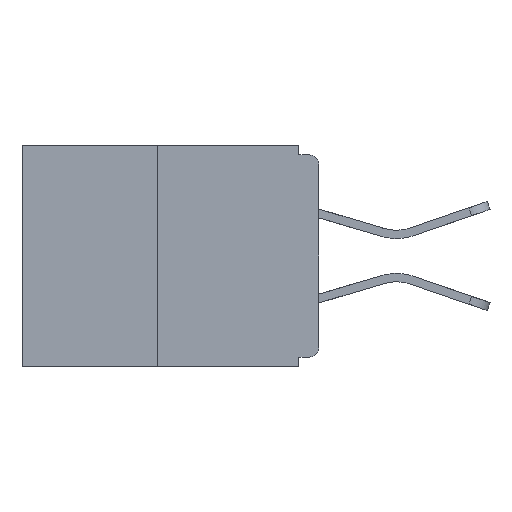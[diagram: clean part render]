
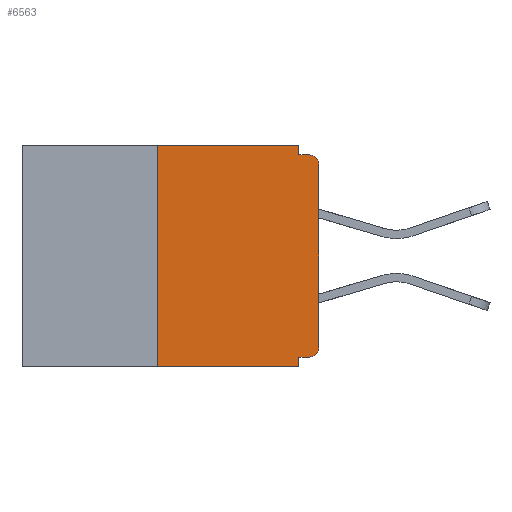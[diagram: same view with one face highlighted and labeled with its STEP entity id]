
A CAD part, left-side view. The second image highlights one B-rep face of the part: STEP entity #6563.
In plain terms, the highlighted planar face has unit normal (-1, 0, 0).
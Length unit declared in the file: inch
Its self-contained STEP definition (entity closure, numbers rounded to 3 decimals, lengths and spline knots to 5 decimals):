
#15 = VERTEX_POINT ( 'NONE', #8032 ) ;
#346 = EDGE_LOOP ( 'NONE', ( #6281, #9837, #14227, #1172, #9857, #2990, #5689, #12049, #8460, #6140 ) ) ;
#632 = VERTEX_POINT ( 'NONE', #10994 ) ;
#756 = VECTOR ( 'NONE', #11183, 39.37008 ) ;
#832 = CARTESIAN_POINT ( 'NONE',  ( 0., 0.25, 0. ) ) ;
#972 = AXIS2_PLACEMENT_3D ( 'NONE', #11592, #3609, #3659 ) ;
#1172 = ORIENTED_EDGE ( 'NONE', *, *, #12081, .F. ) ;
#1865 = DIRECTION ( 'NONE',  ( 0., 0., 1. ) ) ;
#2421 = DIRECTION ( 'NONE',  ( 0., 0., -1. ) ) ;
#2619 = CARTESIAN_POINT ( 'NONE',  ( 0., 0.46, 0. ) ) ;
#2790 = CARTESIAN_POINT ( 'NONE',  ( 0., 0., -0.015 ) ) ;
#2919 = DIRECTION ( 'NONE',  ( 0., 0., -1. ) ) ;
#2990 = ORIENTED_EDGE ( 'NONE', *, *, #7200, .T. ) ;
#3054 = CARTESIAN_POINT ( 'NONE',  ( 0., 0.031, -0.343 ) ) ;
#3356 = VECTOR ( 'NONE', #10710, 39.37008 ) ;
#3609 = DIRECTION ( 'NONE',  ( -1., 0., 0. ) ) ;
#3659 = DIRECTION ( 'NONE',  ( 0., 0., -1. ) ) ;
#4437 = CARTESIAN_POINT ( 'NONE',  ( 0., 0., -0.328 ) ) ;
#4690 = VECTOR ( 'NONE', #11553, 39.37008 ) ;
#4757 = CARTESIAN_POINT ( 'NONE',  ( 0., 0.031, 0. ) ) ;
#4964 = CARTESIAN_POINT ( 'NONE',  ( 0., 0.25, 0. ) ) ;
#5060 = LINE ( 'NONE', #3054, #14374 ) ;
#5541 = DIRECTION ( 'NONE',  ( 0., 0., -1. ) ) ;
#5686 = FACE_OUTER_BOUND ( 'NONE', #346, .T. ) ;
#5689 = ORIENTED_EDGE ( 'NONE', *, *, #9152, .T. ) ;
#5691 = LINE ( 'NONE', #4437, #756 ) ;
#6051 = LINE ( 'NONE', #13934, #4690 ) ;
#6140 = ORIENTED_EDGE ( 'NONE', *, *, #9027, .F. ) ;
#6281 = ORIENTED_EDGE ( 'NONE', *, *, #13015, .F. ) ;
#6563 = ADVANCED_FACE ( 'NONE', ( #5686 ), #8197, .F. ) ;
#6576 = EDGE_CURVE ( 'NONE', #11286, #8579, #7793, .T. ) ;
#6597 = VECTOR ( 'NONE', #14236, 39.37008 ) ;
#6606 = CARTESIAN_POINT ( 'NONE',  ( 0., 0.015, -0.313 ) ) ;
#7036 = CARTESIAN_POINT ( 'NONE',  ( 0., 0., -0.03 ) ) ;
#7200 = EDGE_CURVE ( 'NONE', #15, #9522, #8817, .T. ) ;
#7513 = VECTOR ( 'NONE', #11792, 39.37008 ) ;
#7571 = VERTEX_POINT ( 'NONE', #11605 ) ;
#7793 = CIRCLE ( 'NONE', #972, 0.015 ) ;
#7795 = VERTEX_POINT ( 'NONE', #832 ) ;
#7829 = DIRECTION ( 'NONE',  ( -1., 0., 0. ) ) ;
#8032 = CARTESIAN_POINT ( 'NONE',  ( 0., 0.015, -0.328 ) ) ;
#8197 = PLANE ( 'NONE',  #13336 ) ;
#8452 = EDGE_CURVE ( 'NONE', #7571, #8579, #9648, .T. ) ;
#8460 = ORIENTED_EDGE ( 'NONE', *, *, #8452, .F. ) ;
#8579 = VERTEX_POINT ( 'NONE', #9806 ) ;
#8817 = CIRCLE ( 'NONE', #10686, 0.015 ) ;
#9027 = EDGE_CURVE ( 'NONE', #9532, #7571, #13528, .T. ) ;
#9152 = EDGE_CURVE ( 'NONE', #9522, #11286, #9793, .T. ) ;
#9522 = VERTEX_POINT ( 'NONE', #11418 ) ;
#9532 = VERTEX_POINT ( 'NONE', #4757 ) ;
#9648 = LINE ( 'NONE', #2790, #3356 ) ;
#9793 = LINE ( 'NONE', #13175, #10863 ) ;
#9806 = CARTESIAN_POINT ( 'NONE',  ( 0., 0.015, -0.015 ) ) ;
#9837 = ORIENTED_EDGE ( 'NONE', *, *, #10060, .F. ) ;
#9857 = ORIENTED_EDGE ( 'NONE', *, *, #13605, .F. ) ;
#10060 = EDGE_CURVE ( 'NONE', #14033, #7795, #13702, .T. ) ;
#10150 = EDGE_CURVE ( 'NONE', #14033, #632, #10987, .T. ) ;
#10682 = VECTOR ( 'NONE', #12919, 39.37008 ) ;
#10686 = AXIS2_PLACEMENT_3D ( 'NONE', #6606, #7829, #5541 ) ;
#10710 = DIRECTION ( 'NONE',  ( 0., -1., 0. ) ) ;
#10863 = VECTOR ( 'NONE', #1865, 39.37008 ) ;
#10949 = VERTEX_POINT ( 'NONE', #11134 ) ;
#10987 = LINE ( 'NONE', #11722, #6597 ) ;
#10994 = CARTESIAN_POINT ( 'NONE',  ( 0., 0.031, -0.343 ) ) ;
#11134 = CARTESIAN_POINT ( 'NONE',  ( 0., 0.031, -0.328 ) ) ;
#11183 = DIRECTION ( 'NONE',  ( 0., 1., 0. ) ) ;
#11286 = VERTEX_POINT ( 'NONE', #7036 ) ;
#11418 = CARTESIAN_POINT ( 'NONE',  ( 0., 0., -0.313 ) ) ;
#11459 = DIRECTION ( 'NONE',  ( 1., 0., 0. ) ) ;
#11553 = DIRECTION ( 'NONE',  ( 0., -1., 0. ) ) ;
#11592 = CARTESIAN_POINT ( 'NONE',  ( 0., 0.015, -0.03 ) ) ;
#11605 = CARTESIAN_POINT ( 'NONE',  ( 0., 0.031, -0.015 ) ) ;
#11722 = CARTESIAN_POINT ( 'NONE',  ( 0., 0.46, -0.343 ) ) ;
#11792 = DIRECTION ( 'NONE',  ( 0., 0., -1. ) ) ;
#12049 = ORIENTED_EDGE ( 'NONE', *, *, #6576, .T. ) ;
#12081 = EDGE_CURVE ( 'NONE', #10949, #632, #5060, .T. ) ;
#12892 = CARTESIAN_POINT ( 'NONE',  ( 0., 0.031, 0. ) ) ;
#12919 = DIRECTION ( 'NONE',  ( 0., 0., 1. ) ) ;
#13015 = EDGE_CURVE ( 'NONE', #7795, #9532, #6051, .T. ) ;
#13126 = CARTESIAN_POINT ( 'NONE',  ( 0., 0.25, -0.343 ) ) ;
#13175 = CARTESIAN_POINT ( 'NONE',  ( 0., 0., 0. ) ) ;
#13336 = AXIS2_PLACEMENT_3D ( 'NONE', #2619, #11459, #2421 ) ;
#13528 = LINE ( 'NONE', #12892, #7513 ) ;
#13605 = EDGE_CURVE ( 'NONE', #15, #10949, #5691, .T. ) ;
#13702 = LINE ( 'NONE', #4964, #10682 ) ;
#13934 = CARTESIAN_POINT ( 'NONE',  ( 0., 0.46, 0. ) ) ;
#14033 = VERTEX_POINT ( 'NONE', #13126 ) ;
#14227 = ORIENTED_EDGE ( 'NONE', *, *, #10150, .T. ) ;
#14236 = DIRECTION ( 'NONE',  ( 0., -1., 0. ) ) ;
#14374 = VECTOR ( 'NONE', #2919, 39.37008 ) ;
